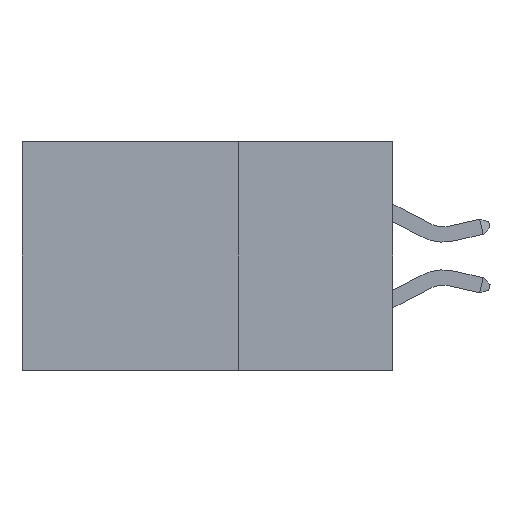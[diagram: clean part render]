
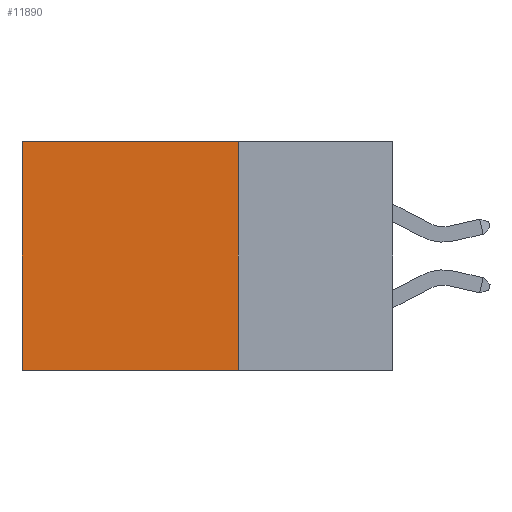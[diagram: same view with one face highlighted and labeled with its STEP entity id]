
A CAD part, left-side view. The second image highlights one B-rep face of the part: STEP entity #11890.
In plain terms, the highlighted planar face has unit normal (-1, 0, 0).
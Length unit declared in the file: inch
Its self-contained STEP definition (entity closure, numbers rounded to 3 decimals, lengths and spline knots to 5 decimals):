
#341 = EDGE_CURVE ( 'NONE', #15526, #8085, #16337, .T. ) ;
#587 = DIRECTION ( 'NONE',  ( 0., 0., -1. ) ) ;
#1960 = CARTESIAN_POINT ( 'NONE',  ( 0.2875, 0.6, 0. ) ) ;
#2157 = DIRECTION ( 'NONE',  ( 0., 0., -1. ) ) ;
#2797 = ORIENTED_EDGE ( 'NONE', *, *, #6332, .T. ) ;
#2929 = AXIS2_PLACEMENT_3D ( 'NONE', #7132, #8397, #587 ) ;
#3214 = LINE ( 'NONE', #11236, #16529 ) ;
#4112 = CARTESIAN_POINT ( 'NONE',  ( 0.2875, 0.25, -0.37 ) ) ;
#4331 = VERTEX_POINT ( 'NONE', #11866 ) ;
#6292 = VECTOR ( 'NONE', #14717, 39.37008 ) ;
#6332 = EDGE_CURVE ( 'NONE', #11156, #8085, #10060, .T. ) ;
#6591 = EDGE_LOOP ( 'NONE', ( #2797, #7432, #14214, #12645 ) ) ;
#6934 = DIRECTION ( 'NONE',  ( 0., 1., 0. ) ) ;
#7132 = CARTESIAN_POINT ( 'NONE',  ( 0.2875, 0.25, 0. ) ) ;
#7432 = ORIENTED_EDGE ( 'NONE', *, *, #341, .F. ) ;
#7543 = CARTESIAN_POINT ( 'NONE',  ( 0.2875, 0.6, 0. ) ) ;
#8085 = VERTEX_POINT ( 'NONE', #15201 ) ;
#8264 = CARTESIAN_POINT ( 'NONE',  ( 0.2875, 0.25, 0. ) ) ;
#8397 = DIRECTION ( 'NONE',  ( 1., 0., 0. ) ) ;
#10060 = LINE ( 'NONE', #7543, #12326 ) ;
#10134 = VECTOR ( 'NONE', #6934, 39.37008 ) ;
#10445 = FACE_OUTER_BOUND ( 'NONE', #6591, .T. ) ;
#11156 = VERTEX_POINT ( 'NONE', #1960 ) ;
#11236 = CARTESIAN_POINT ( 'NONE',  ( 0.2875, 0.25, 0. ) ) ;
#11598 = LINE ( 'NONE', #8264, #10134 ) ;
#11866 = CARTESIAN_POINT ( 'NONE',  ( 0.2875, 0.25, 0. ) ) ;
#11890 = ADVANCED_FACE ( 'NONE', ( #10445 ), #13662, .F. ) ;
#11936 = CARTESIAN_POINT ( 'NONE',  ( 0.2875, 0.25, -0.37 ) ) ;
#12326 = VECTOR ( 'NONE', #2157, 39.37008 ) ;
#12645 = ORIENTED_EDGE ( 'NONE', *, *, #13570, .T. ) ;
#13570 = EDGE_CURVE ( 'NONE', #4331, #11156, #11598, .T. ) ;
#13662 = PLANE ( 'NONE',  #2929 ) ;
#13772 = DIRECTION ( 'NONE',  ( 0., 0., -1. ) ) ;
#14214 = ORIENTED_EDGE ( 'NONE', *, *, #16052, .F. ) ;
#14717 = DIRECTION ( 'NONE',  ( 0., 1., 0. ) ) ;
#15201 = CARTESIAN_POINT ( 'NONE',  ( 0.2875, 0.6, -0.37 ) ) ;
#15526 = VERTEX_POINT ( 'NONE', #11936 ) ;
#16052 = EDGE_CURVE ( 'NONE', #4331, #15526, #3214, .T. ) ;
#16337 = LINE ( 'NONE', #4112, #6292 ) ;
#16529 = VECTOR ( 'NONE', #13772, 39.37008 ) ;
